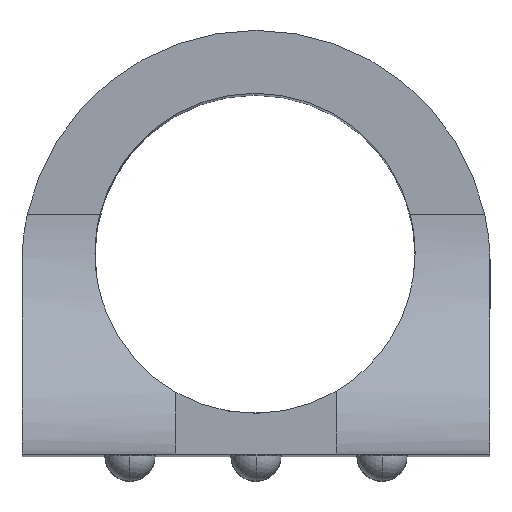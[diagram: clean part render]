
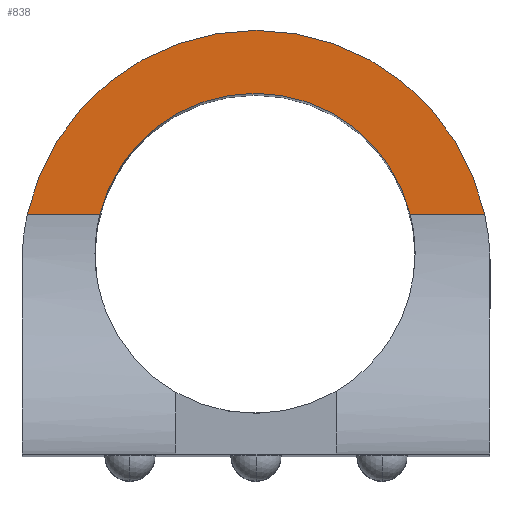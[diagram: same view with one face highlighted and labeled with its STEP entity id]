
A CAD part, top view. The second image highlights one B-rep face of the part: STEP entity #838.
In plain terms, the highlighted planar face has unit normal (0, 0, 1).
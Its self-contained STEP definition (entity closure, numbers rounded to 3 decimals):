
#55 = EDGE_CURVE ( 'NONE', #1681, #1598, #1587, .T. ) ;
#73 = CARTESIAN_POINT ( 'NONE',  ( 19.419, 43.328, -15.408 ) ) ;
#80 = EDGE_CURVE ( 'NONE', #1681, #272, #340, .T. ) ;
#99 = DIRECTION ( 'NONE',  ( 0., 0., 1. ) ) ;
#177 = DIRECTION ( 'NONE',  ( 1., 0., 0. ) ) ;
#217 = DIRECTION ( 'NONE',  ( 1., 0., 0. ) ) ;
#228 = EDGE_CURVE ( 'NONE', #1518, #1598, #1235, .T. ) ;
#272 = VERTEX_POINT ( 'NONE', #1540 ) ;
#315 = EDGE_CURVE ( 'NONE', #1518, #272, #1140, .T. ) ;
#340 = LINE ( 'NONE', #873, #1151 ) ;
#387 = AXIS2_PLACEMENT_3D ( 'NONE', #868, #99, #217 ) ;
#422 = CARTESIAN_POINT ( 'NONE',  ( 44.058, 43.328, -15.408 ) ) ;
#547 = VECTOR ( 'NONE', #1245, 1000. ) ;
#592 = ORIENTED_EDGE ( 'NONE', *, *, #228, .F. ) ;
#595 = DIRECTION ( 'NONE',  ( -1., 0., 0. ) ) ;
#713 = CARTESIAN_POINT ( 'NONE',  ( 49.961, 43.328, -15.408 ) ) ;
#762 = DIRECTION ( 'NONE',  ( 1., 0., 0. ) ) ;
#838 = ADVANCED_FACE ( 'NONE', ( #1714 ), #1553, .T. ) ;
#854 = CARTESIAN_POINT ( 'NONE',  ( 31.739, 40.242, -15.408 ) ) ;
#868 = CARTESIAN_POINT ( 'NONE',  ( 31.815, 39.361, -15.408 ) ) ;
#873 = CARTESIAN_POINT ( 'NONE',  ( 19.419, 43.328, -15.408 ) ) ;
#881 = AXIS2_PLACEMENT_3D ( 'NONE', #896, #1310, #762 ) ;
#896 = CARTESIAN_POINT ( 'NONE',  ( 50.382, 17.915, -15.408 ) ) ;
#907 = ORIENTED_EDGE ( 'NONE', *, *, #315, .T. ) ;
#1140 = CIRCLE ( 'NONE', #387, 18.575 ) ;
#1151 = VECTOR ( 'NONE', #595, 1000. ) ;
#1190 = CARTESIAN_POINT ( 'NONE',  ( 49.961, 43.328, -15.408 ) ) ;
#1235 = LINE ( 'NONE', #713, #547 ) ;
#1245 = DIRECTION ( 'NONE',  ( -1., 0., 0. ) ) ;
#1253 = ORIENTED_EDGE ( 'NONE', *, *, #55, .T. ) ;
#1258 = EDGE_LOOP ( 'NONE', ( #592, #907, #1350, #1253 ) ) ;
#1310 = DIRECTION ( 'NONE',  ( 0., 0., 1. ) ) ;
#1350 = ORIENTED_EDGE ( 'NONE', *, *, #80, .F. ) ;
#1360 = DIRECTION ( 'NONE',  ( 0., 0., -1. ) ) ;
#1372 = AXIS2_PLACEMENT_3D ( 'NONE', #854, #1360, #177 ) ;
#1518 = VERTEX_POINT ( 'NONE', #1190 ) ;
#1540 = CARTESIAN_POINT ( 'NONE',  ( 13.668, 43.328, -15.408 ) ) ;
#1553 = PLANE ( 'NONE',  #881 ) ;
#1587 = CIRCLE ( 'NONE', #1372, 12.7 ) ;
#1598 = VERTEX_POINT ( 'NONE', #422 ) ;
#1681 = VERTEX_POINT ( 'NONE', #73 ) ;
#1714 = FACE_OUTER_BOUND ( 'NONE', #1258, .T. ) ;
